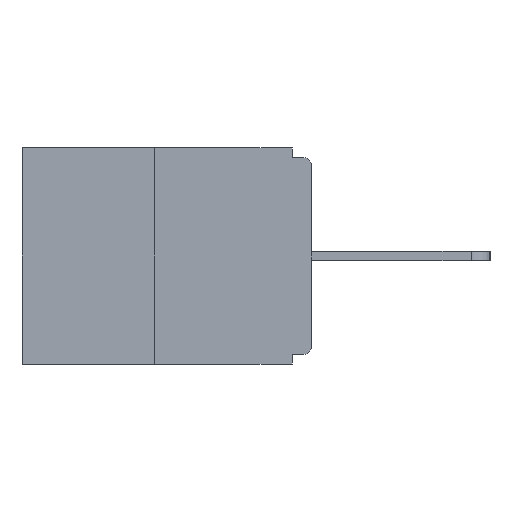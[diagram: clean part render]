
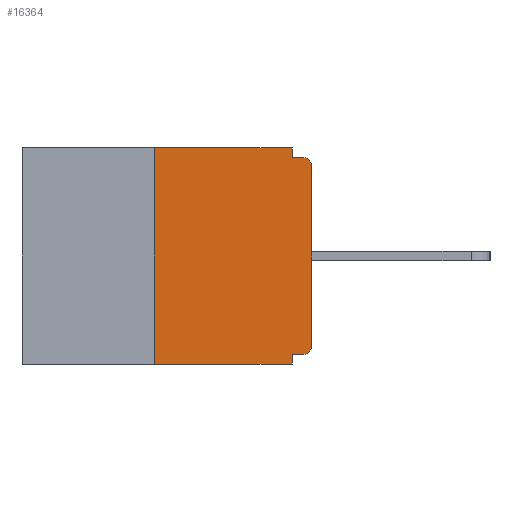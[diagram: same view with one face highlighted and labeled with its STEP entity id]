
A CAD part, left-side view. The second image highlights one B-rep face of the part: STEP entity #16364.
In plain terms, the highlighted planar face has unit normal (-1, 0, 0).
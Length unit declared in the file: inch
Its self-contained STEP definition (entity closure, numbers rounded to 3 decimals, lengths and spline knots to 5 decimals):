
#295 = CARTESIAN_POINT ( 'NONE',  ( 0., 0.25, 0. ) ) ;
#1311 = CARTESIAN_POINT ( 'NONE',  ( 0., 0., 0. ) ) ;
#1440 = CIRCLE ( 'NONE', #18677, 0.015 ) ;
#1563 = DIRECTION ( 'NONE',  ( 0., 0., -1. ) ) ;
#2064 = VECTOR ( 'NONE', #26220, 39.37008 ) ;
#2442 = DIRECTION ( 'NONE',  ( 0., 0., 1. ) ) ;
#2662 = EDGE_CURVE ( 'NONE', #4049, #22921, #1440, .T. ) ;
#3168 = CARTESIAN_POINT ( 'NONE',  ( 0., 0.25, -0.343 ) ) ;
#3179 = VERTEX_POINT ( 'NONE', #20032 ) ;
#3274 = CARTESIAN_POINT ( 'NONE',  ( 0., 0.031, -0.343 ) ) ;
#3512 = CARTESIAN_POINT ( 'NONE',  ( 0., 0.46, 0. ) ) ;
#3896 = CIRCLE ( 'NONE', #19341, 0.015 ) ;
#4026 = LINE ( 'NONE', #26224, #25003 ) ;
#4049 = VERTEX_POINT ( 'NONE', #22425 ) ;
#4063 = DIRECTION ( 'NONE',  ( -1., 0., 0. ) ) ;
#4255 = EDGE_CURVE ( 'NONE', #10358, #11815, #4026, .T. ) ;
#4460 = DIRECTION ( 'NONE',  ( 0., -1., 0. ) ) ;
#4721 = VERTEX_POINT ( 'NONE', #3274 ) ;
#4999 = EDGE_CURVE ( 'NONE', #22921, #8797, #24168, .T. ) ;
#5054 = CARTESIAN_POINT ( 'NONE',  ( 0., 0.46, -0.343 ) ) ;
#5688 = EDGE_CURVE ( 'NONE', #3179, #4721, #7715, .T. ) ;
#5872 = LINE ( 'NONE', #24326, #16916 ) ;
#6374 = DIRECTION ( 'NONE',  ( 0., 0., 1. ) ) ;
#6387 = FACE_OUTER_BOUND ( 'NONE', #15252, .T. ) ;
#6560 = ORIENTED_EDGE ( 'NONE', *, *, #25014, .T. ) ;
#7100 = EDGE_CURVE ( 'NONE', #14711, #4721, #21944, .T. ) ;
#7419 = VECTOR ( 'NONE', #6374, 39.37008 ) ;
#7715 = LINE ( 'NONE', #9036, #2064 ) ;
#8114 = VECTOR ( 'NONE', #11864, 39.37008 ) ;
#8797 = VERTEX_POINT ( 'NONE', #10877 ) ;
#9036 = CARTESIAN_POINT ( 'NONE',  ( 0., 0.031, -0.343 ) ) ;
#9901 = PLANE ( 'NONE',  #17082 ) ;
#9968 = LINE ( 'NONE', #19896, #14813 ) ;
#10358 = VERTEX_POINT ( 'NONE', #11280 ) ;
#10877 = CARTESIAN_POINT ( 'NONE',  ( 0., 0., -0.03 ) ) ;
#11208 = EDGE_CURVE ( 'NONE', #11815, #25848, #9968, .T. ) ;
#11280 = CARTESIAN_POINT ( 'NONE',  ( 0., 0.031, 0. ) ) ;
#11531 = ORIENTED_EDGE ( 'NONE', *, *, #2662, .T. ) ;
#11689 = CARTESIAN_POINT ( 'NONE',  ( 0., 0.015, -0.313 ) ) ;
#11815 = VERTEX_POINT ( 'NONE', #21740 ) ;
#11864 = DIRECTION ( 'NONE',  ( 0., 1., 0. ) ) ;
#11901 = ORIENTED_EDGE ( 'NONE', *, *, #20664, .F. ) ;
#11964 = ORIENTED_EDGE ( 'NONE', *, *, #5688, .F. ) ;
#12052 = DIRECTION ( 'NONE',  ( 0., 0., -1. ) ) ;
#12082 = CARTESIAN_POINT ( 'NONE',  ( 0., 0.25, 0. ) ) ;
#12427 = LINE ( 'NONE', #25722, #8114 ) ;
#12469 = DIRECTION ( 'NONE',  ( 0., -1., 0. ) ) ;
#12767 = EDGE_CURVE ( 'NONE', #14711, #15739, #16950, .T. ) ;
#13336 = DIRECTION ( 'NONE',  ( -1., 0., 0. ) ) ;
#13676 = DIRECTION ( 'NONE',  ( 0., 0., -1. ) ) ;
#14711 = VERTEX_POINT ( 'NONE', #3168 ) ;
#14813 = VECTOR ( 'NONE', #25746, 39.37008 ) ;
#15252 = EDGE_LOOP ( 'NONE', ( #25156, #19763, #19045, #11964, #11901, #11531, #18193, #6560, #19123, #21287 ) ) ;
#15739 = VERTEX_POINT ( 'NONE', #12082 ) ;
#16364 = ADVANCED_FACE ( 'NONE', ( #6387 ), #9901, .F. ) ;
#16572 = CARTESIAN_POINT ( 'NONE',  ( 0., 0.015, -0.03 ) ) ;
#16702 = VECTOR ( 'NONE', #4460, 39.37008 ) ;
#16916 = VECTOR ( 'NONE', #12469, 39.37008 ) ;
#16950 = LINE ( 'NONE', #295, #20701 ) ;
#17082 = AXIS2_PLACEMENT_3D ( 'NONE', #3512, #23939, #12052 ) ;
#18193 = ORIENTED_EDGE ( 'NONE', *, *, #4999, .T. ) ;
#18557 = DIRECTION ( 'NONE',  ( 0., 0., -1. ) ) ;
#18677 = AXIS2_PLACEMENT_3D ( 'NONE', #11689, #13336, #13676 ) ;
#19045 = ORIENTED_EDGE ( 'NONE', *, *, #7100, .T. ) ;
#19123 = ORIENTED_EDGE ( 'NONE', *, *, #11208, .F. ) ;
#19341 = AXIS2_PLACEMENT_3D ( 'NONE', #16572, #4063, #18557 ) ;
#19625 = EDGE_CURVE ( 'NONE', #15739, #10358, #5872, .T. ) ;
#19763 = ORIENTED_EDGE ( 'NONE', *, *, #12767, .F. ) ;
#19896 = CARTESIAN_POINT ( 'NONE',  ( 0., 0., -0.015 ) ) ;
#20032 = CARTESIAN_POINT ( 'NONE',  ( 0., 0.031, -0.328 ) ) ;
#20664 = EDGE_CURVE ( 'NONE', #4049, #3179, #12427, .T. ) ;
#20701 = VECTOR ( 'NONE', #2442, 39.37008 ) ;
#21195 = CARTESIAN_POINT ( 'NONE',  ( 0., 0.015, -0.015 ) ) ;
#21287 = ORIENTED_EDGE ( 'NONE', *, *, #4255, .F. ) ;
#21740 = CARTESIAN_POINT ( 'NONE',  ( 0., 0.031, -0.015 ) ) ;
#21944 = LINE ( 'NONE', #5054, #16702 ) ;
#22302 = CARTESIAN_POINT ( 'NONE',  ( 0., 0., -0.313 ) ) ;
#22425 = CARTESIAN_POINT ( 'NONE',  ( 0., 0.015, -0.328 ) ) ;
#22921 = VERTEX_POINT ( 'NONE', #22302 ) ;
#23939 = DIRECTION ( 'NONE',  ( 1., 0., 0. ) ) ;
#24168 = LINE ( 'NONE', #1311, #7419 ) ;
#24326 = CARTESIAN_POINT ( 'NONE',  ( 0., 0.46, 0. ) ) ;
#25003 = VECTOR ( 'NONE', #1563, 39.37008 ) ;
#25014 = EDGE_CURVE ( 'NONE', #8797, #25848, #3896, .T. ) ;
#25156 = ORIENTED_EDGE ( 'NONE', *, *, #19625, .F. ) ;
#25722 = CARTESIAN_POINT ( 'NONE',  ( 0., 0., -0.328 ) ) ;
#25746 = DIRECTION ( 'NONE',  ( 0., -1., 0. ) ) ;
#25848 = VERTEX_POINT ( 'NONE', #21195 ) ;
#26220 = DIRECTION ( 'NONE',  ( 0., 0., -1. ) ) ;
#26224 = CARTESIAN_POINT ( 'NONE',  ( 0., 0.031, 0. ) ) ;
